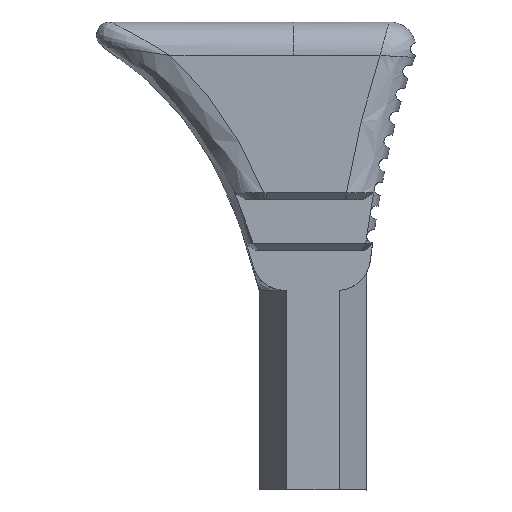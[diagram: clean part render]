
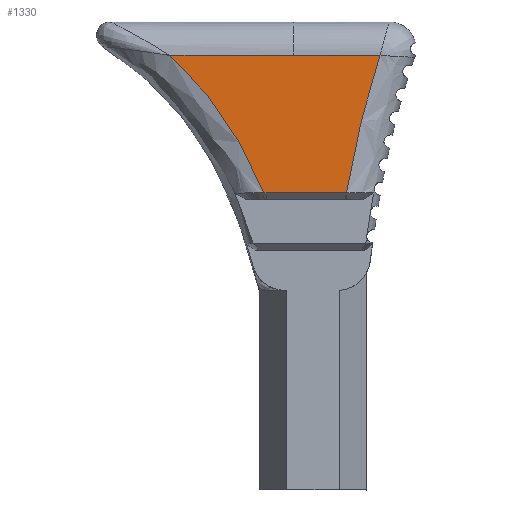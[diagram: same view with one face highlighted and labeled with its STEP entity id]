
A CAD part, top view. The second image highlights one B-rep face of the part: STEP entity #1330.
In plain terms, the highlighted planar face has unit normal (0, 0, 1).
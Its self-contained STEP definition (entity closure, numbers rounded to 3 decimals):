
#65=PLANE('',#1408);
#100=FACE_OUTER_BOUND('',#178,.T.);
#178=EDGE_LOOP('',(#942,#943,#944,#945,#946,#947,#948));
#250=LINE('',#2437,#299);
#254=LINE('',#2555,#303);
#255=LINE('',#2556,#304);
#299=VECTOR('',#1480,10.);
#303=VECTOR('',#1486,10.);
#304=VECTOR('',#1487,10.);
#368=B_SPLINE_CURVE_WITH_KNOTS('',3,(#2165,#2166,#2167,#2168,#2169,#2170,
#2171,#2172,#2173,#2174),.UNSPECIFIED.,.F.,.F.,(4,3,3,4),(-1.708,
-1.169,-0.584,-0.458),.UNSPECIFIED.);
#386=B_SPLINE_CURVE_WITH_KNOTS('',3,(#2457,#2458,#2459,#2460),
 .UNSPECIFIED.,.F.,.F.,(4,4),(0.,0.02),.UNSPECIFIED.);
#390=B_SPLINE_CURVE_WITH_KNOTS('',3,(#2540,#2541,#2542,#2543),
 .UNSPECIFIED.,.F.,.F.,(4,4),(0.285,0.293),
 .UNSPECIFIED.);
#392=B_SPLINE_CURVE_WITH_KNOTS('',3,(#2550,#2551,#2552,#2553),
 .UNSPECIFIED.,.F.,.F.,(4,4),(0.07,1.123),
 .UNSPECIFIED.);
#512=VERTEX_POINT('',#2153);
#513=VERTEX_POINT('',#2164);
#531=VERTEX_POINT('',#2434);
#532=VERTEX_POINT('',#2436);
#534=VERTEX_POINT('',#2505);
#536=VERTEX_POINT('',#2549);
#537=VERTEX_POINT('',#2554);
#662=EDGE_CURVE('',#512,#513,#368,.T.);
#686=EDGE_CURVE('',#531,#532,#250,.T.);
#689=EDGE_CURVE('',#532,#512,#386,.T.);
#694=EDGE_CURVE('',#534,#531,#390,.T.);
#696=EDGE_CURVE('',#536,#534,#392,.T.);
#697=EDGE_CURVE('',#537,#536,#254,.T.);
#698=EDGE_CURVE('',#513,#537,#255,.T.);
#942=ORIENTED_EDGE('',*,*,#689,.F.);
#943=ORIENTED_EDGE('',*,*,#686,.F.);
#944=ORIENTED_EDGE('',*,*,#694,.F.);
#945=ORIENTED_EDGE('',*,*,#696,.F.);
#946=ORIENTED_EDGE('',*,*,#697,.F.);
#947=ORIENTED_EDGE('',*,*,#698,.F.);
#948=ORIENTED_EDGE('',*,*,#662,.F.);
#1330=ADVANCED_FACE('',(#100),#65,.F.);
#1408=AXIS2_PLACEMENT_3D('',#2548,#1484,#1485);
#1480=DIRECTION('',(-1.,0.,0.));
#1484=DIRECTION('center_axis',(0.,0.,
-1.));
#1485=DIRECTION('ref_axis',(-1.,0.,0.));
#1486=DIRECTION('',(1.,0.,0.));
#1487=DIRECTION('',(1.,0.,0.));
#2153=CARTESIAN_POINT('',(2853.896,486.942,126.567));
#2164=CARTESIAN_POINT('',(2846.917,497.176,126.567));
#2165=CARTESIAN_POINT('Ctrl Pts',(2853.897,486.947,126.567));
#2166=CARTESIAN_POINT('Ctrl Pts',(2853.219,488.611,126.567));
#2167=CARTESIAN_POINT('Ctrl Pts',(2852.419,490.226,126.567));
#2168=CARTESIAN_POINT('Ctrl Pts',(2851.466,491.748,126.567));
#2169=CARTESIAN_POINT('Ctrl Pts',(2850.432,493.398,126.567));
#2170=CARTESIAN_POINT('Ctrl Pts',(2849.216,494.939,126.567));
#2171=CARTESIAN_POINT('Ctrl Pts',(2847.836,496.312,126.567));
#2172=CARTESIAN_POINT('Ctrl Pts',(2847.538,496.609,126.567));
#2173=CARTESIAN_POINT('Ctrl Pts',(2847.233,496.897,126.567));
#2174=CARTESIAN_POINT('Ctrl Pts',(2846.92,497.178,126.567));
#2434=CARTESIAN_POINT('',(2859.985,486.942,126.567));
#2436=CARTESIAN_POINT('',(2854.097,486.942,126.567));
#2437=CARTESIAN_POINT('',(2849.88,486.942,126.567));
#2457=CARTESIAN_POINT('Ctrl Pts',(2854.097,486.942,126.567));
#2458=CARTESIAN_POINT('Ctrl Pts',(2854.03,486.942,126.567));
#2459=CARTESIAN_POINT('Ctrl Pts',(2853.963,486.942,126.567));
#2460=CARTESIAN_POINT('Ctrl Pts',(2853.896,486.942,126.567));
#2505=CARTESIAN_POINT('',(2860.069,486.942,126.567));
#2540=CARTESIAN_POINT('Ctrl Pts',(2860.069,486.942,126.567));
#2541=CARTESIAN_POINT('Ctrl Pts',(2860.041,486.942,126.567));
#2542=CARTESIAN_POINT('Ctrl Pts',(2860.013,486.942,126.567));
#2543=CARTESIAN_POINT('Ctrl Pts',(2859.985,486.942,126.567));
#2548=CARTESIAN_POINT('Origin',(2849.721,489.676,126.567));
#2549=CARTESIAN_POINT('',(2862.559,497.176,126.567));
#2550=CARTESIAN_POINT('Ctrl Pts',(2862.559,497.176,126.567));
#2551=CARTESIAN_POINT('Ctrl Pts',(2861.468,493.838,126.567));
#2552=CARTESIAN_POINT('Ctrl Pts',(2860.668,490.406,126.567));
#2553=CARTESIAN_POINT('Ctrl Pts',(2860.07,486.942,126.567));
#2554=CARTESIAN_POINT('',(2856.11,497.176,126.567));
#2555=CARTESIAN_POINT('',(2854.379,497.176,126.567));
#2556=CARTESIAN_POINT('',(2851.647,497.176,126.567));
